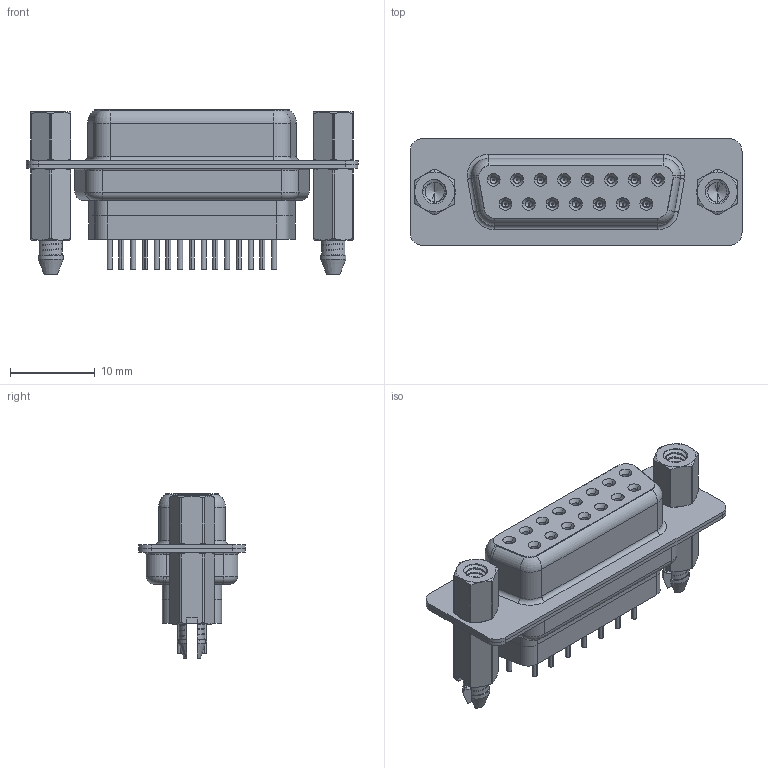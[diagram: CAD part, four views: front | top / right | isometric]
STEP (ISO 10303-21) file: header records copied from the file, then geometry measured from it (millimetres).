
FILE_DESCRIPTION (( 'STEP AP203' ), '1' );
FILE_NAME ('628-015-228-267.STEP', '2020-07-21T13:31:26', ( '' ), ( '' ), 'SwSTEP 2.0', 'SolidWorks 2020', '' );
FILE_SCHEMA (( 'CONFIG_CONTROL_DESIGN' ));
Length unit declared in the file: millimetre
Products named in the file (8): 628 Housing_15 FF; 628 4-40 Threaded Boardlock_FF; 628 Contact Row 2_28L; 628 4-40 Hex Standoff; 628 Shell Rear_15 Contacts; 628 Shell Front_15 Contacts; 628-015-228-267; 628 Contact Row 1_28L
Assembly tree (22 placements, depth 2):
  628-015-228-267
    628 Housing_15 FF
    628 Shell Front_15 Contacts
    628 Shell Rear_15 Contacts
    628 Contact Row 1_28L  x8
    628 Contact Row 2_28L  x7
    628 4-40 Hex Standoff  x2
    628 4-40 Threaded Boardlock_FF  x2
Bounding box: 39.15 x 12.6 x 19.4 mm (x, y, z)
Volume: 3310 mm3; surface area: 7984.2 mm2
Topology: 23 solids, 23 shells, 2507 faces, 6482 edges, 4060 vertices
Faces by surface type: cylinder 805, plane 592, torus 453, bspline 366, cone 291
Entity records: 46473 total; most frequent: CARTESIAN_POINT 25335, ORIENTED_EDGE 4262, DIRECTION 4116, EDGE_CURVE 2131, AXIS2_PLACEMENT_3D 1683, VERTEX_POINT 1355, EDGE_LOOP 976, CIRCLE 884
